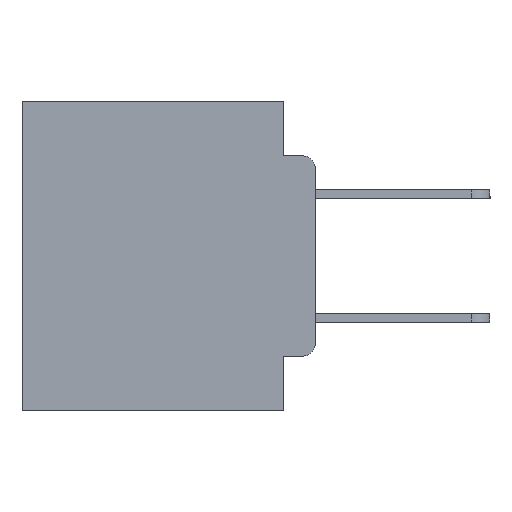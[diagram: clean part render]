
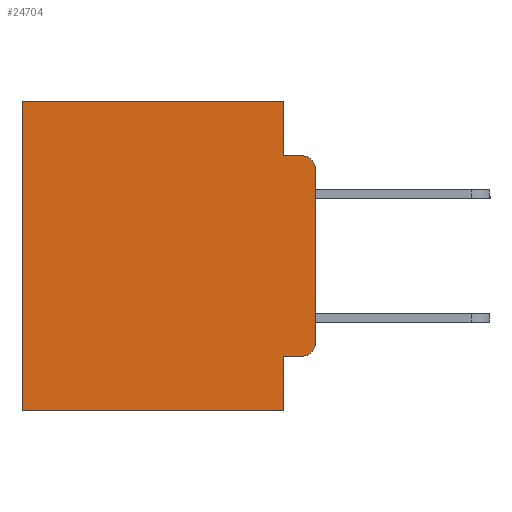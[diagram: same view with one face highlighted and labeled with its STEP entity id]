
A CAD part, left-side view. The second image highlights one B-rep face of the part: STEP entity #24704.
In plain terms, the highlighted planar face has unit normal (-1, 0, 0).
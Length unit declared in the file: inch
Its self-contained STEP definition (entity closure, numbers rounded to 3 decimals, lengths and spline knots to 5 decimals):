
#79 = CARTESIAN_POINT ( 'NONE',  ( 0.298, 0.02, -0.3915 ) ) ;
#469 = DIRECTION ( 'NONE',  ( 0., 1., 0. ) ) ;
#628 = VERTEX_POINT ( 'NONE', #25031 ) ;
#673 = ORIENTED_EDGE ( 'NONE', *, *, #13009, .T. ) ;
#2042 = VERTEX_POINT ( 'NONE', #24449 ) ;
#2286 = LINE ( 'NONE', #4082, #17867 ) ;
#2313 = DIRECTION ( 'NONE',  ( 0., 0., -1. ) ) ;
#2381 = AXIS2_PLACEMENT_3D ( 'NONE', #79, #15123, #2313 ) ;
#2742 = ORIENTED_EDGE ( 'NONE', *, *, #22740, .T. ) ;
#2755 = CARTESIAN_POINT ( 'NONE',  ( 0.298, 0.473, 0. ) ) ;
#3149 = CARTESIAN_POINT ( 'NONE',  ( 0.298, 0.051, -0.0885 ) ) ;
#3529 = VERTEX_POINT ( 'NONE', #14324 ) ;
#3605 = DIRECTION ( 'NONE',  ( 0., 0., -1. ) ) ;
#4082 = CARTESIAN_POINT ( 'NONE',  ( 0.298, 0., 0. ) ) ;
#4726 = EDGE_CURVE ( 'NONE', #12603, #23204, #25834, .T. ) ;
#5022 = AXIS2_PLACEMENT_3D ( 'NONE', #22493, #16322, #3605 ) ;
#5217 = ORIENTED_EDGE ( 'NONE', *, *, #4726, .T. ) ;
#5502 = LINE ( 'NONE', #15865, #15423 ) ;
#5717 = CARTESIAN_POINT ( 'NONE',  ( 0.298, 0.02, -0.1085 ) ) ;
#5826 = ORIENTED_EDGE ( 'NONE', *, *, #17916, .T. ) ;
#5910 = CARTESIAN_POINT ( 'NONE',  ( 0.298, 0.02, -0.0885 ) ) ;
#6348 = AXIS2_PLACEMENT_3D ( 'NONE', #5717, #20419, #8233 ) ;
#6948 = ORIENTED_EDGE ( 'NONE', *, *, #24230, .F. ) ;
#7505 = DIRECTION ( 'NONE',  ( 0., -1., 0. ) ) ;
#8233 = DIRECTION ( 'NONE',  ( 0., 0., -1. ) ) ;
#8245 = VECTOR ( 'NONE', #7505, 39.37008 ) ;
#8340 = DIRECTION ( 'NONE',  ( 0., 0., -1. ) ) ;
#8651 = ORIENTED_EDGE ( 'NONE', *, *, #15200, .F. ) ;
#8920 = VECTOR ( 'NONE', #19957, 39.37008 ) ;
#9114 = EDGE_LOOP ( 'NONE', ( #6948, #17652, #15808, #8651, #5217, #5826, #23915, #23700, #2742, #673 ) ) ;
#9290 = VERTEX_POINT ( 'NONE', #16609 ) ;
#9604 = CARTESIAN_POINT ( 'NONE',  ( 0.298, 0.473, 0. ) ) ;
#9780 = FACE_OUTER_BOUND ( 'NONE', #9114, .T. ) ;
#10179 = VECTOR ( 'NONE', #24489, 39.37008 ) ;
#10869 = CARTESIAN_POINT ( 'NONE',  ( 0.298, 0.051, -0.0885 ) ) ;
#12204 = VERTEX_POINT ( 'NONE', #5910 ) ;
#12331 = VERTEX_POINT ( 'NONE', #16849 ) ;
#12603 = VERTEX_POINT ( 'NONE', #13721 ) ;
#12658 = VECTOR ( 'NONE', #26302, 39.37008 ) ;
#13009 = EDGE_CURVE ( 'NONE', #9290, #12331, #16472, .T. ) ;
#13721 = CARTESIAN_POINT ( 'NONE',  ( 0.298, 0.051, 0. ) ) ;
#13828 = EDGE_CURVE ( 'NONE', #27100, #12204, #18033, .T. ) ;
#14053 = CARTESIAN_POINT ( 'NONE',  ( 0.298, 0.051, -0.4115 ) ) ;
#14252 = PLANE ( 'NONE',  #5022 ) ;
#14324 = CARTESIAN_POINT ( 'NONE',  ( 0.298, 0.051, -0.5 ) ) ;
#14757 = VECTOR ( 'NONE', #469, 39.37008 ) ;
#15123 = DIRECTION ( 'NONE',  ( -1., 0., 0. ) ) ;
#15200 = EDGE_CURVE ( 'NONE', #12603, #27100, #5502, .T. ) ;
#15405 = LINE ( 'NONE', #23357, #20268 ) ;
#15423 = VECTOR ( 'NONE', #17892, 39.37008 ) ;
#15744 = LINE ( 'NONE', #14053, #10179 ) ;
#15808 = ORIENTED_EDGE ( 'NONE', *, *, #13828, .F. ) ;
#15865 = CARTESIAN_POINT ( 'NONE',  ( 0.298, 0.051, 0. ) ) ;
#16322 = DIRECTION ( 'NONE',  ( 1., 0., 0. ) ) ;
#16472 = CIRCLE ( 'NONE', #2381, 0.02 ) ;
#16609 = CARTESIAN_POINT ( 'NONE',  ( 0.298, 0.02, -0.4115 ) ) ;
#16849 = CARTESIAN_POINT ( 'NONE',  ( 0.298, 0., -0.3915 ) ) ;
#17513 = CARTESIAN_POINT ( 'NONE',  ( 0.298, 0., 0. ) ) ;
#17652 = ORIENTED_EDGE ( 'NONE', *, *, #20564, .T. ) ;
#17831 = CARTESIAN_POINT ( 'NONE',  ( 0.298, 0.051, 0. ) ) ;
#17867 = VECTOR ( 'NONE', #8340, 39.37008 ) ;
#17892 = DIRECTION ( 'NONE',  ( 0., 0., -1. ) ) ;
#17916 = EDGE_CURVE ( 'NONE', #23204, #2042, #23736, .T. ) ;
#18033 = LINE ( 'NONE', #3149, #8245 ) ;
#19957 = DIRECTION ( 'NONE',  ( 0., 0., -1. ) ) ;
#20268 = VECTOR ( 'NONE', #25458, 39.37008 ) ;
#20419 = DIRECTION ( 'NONE',  ( -1., 0., 0. ) ) ;
#20564 = EDGE_CURVE ( 'NONE', #24206, #12204, #20736, .T. ) ;
#20736 = CIRCLE ( 'NONE', #6348, 0.02 ) ;
#21503 = EDGE_CURVE ( 'NONE', #628, #3529, #25583, .T. ) ;
#22493 = CARTESIAN_POINT ( 'NONE',  ( 0.298, 0., 0. ) ) ;
#22740 = EDGE_CURVE ( 'NONE', #628, #9290, #15744, .T. ) ;
#22961 = CARTESIAN_POINT ( 'NONE',  ( 0.298, 0., -0.1085 ) ) ;
#23016 = EDGE_CURVE ( 'NONE', #3529, #2042, #15405, .T. ) ;
#23204 = VERTEX_POINT ( 'NONE', #2755 ) ;
#23357 = CARTESIAN_POINT ( 'NONE',  ( 0.298, 0., -0.5 ) ) ;
#23700 = ORIENTED_EDGE ( 'NONE', *, *, #21503, .F. ) ;
#23736 = LINE ( 'NONE', #9604, #12658 ) ;
#23915 = ORIENTED_EDGE ( 'NONE', *, *, #23016, .F. ) ;
#24206 = VERTEX_POINT ( 'NONE', #22961 ) ;
#24230 = EDGE_CURVE ( 'NONE', #24206, #12331, #2286, .T. ) ;
#24449 = CARTESIAN_POINT ( 'NONE',  ( 0.298, 0.473, -0.5 ) ) ;
#24489 = DIRECTION ( 'NONE',  ( 0., -1., 0. ) ) ;
#24704 = ADVANCED_FACE ( 'NONE', ( #9780 ), #14252, .F. ) ;
#25031 = CARTESIAN_POINT ( 'NONE',  ( 0.298, 0.051, -0.4115 ) ) ;
#25458 = DIRECTION ( 'NONE',  ( 0., 1., 0. ) ) ;
#25583 = LINE ( 'NONE', #17831, #8920 ) ;
#25834 = LINE ( 'NONE', #17513, #14757 ) ;
#26302 = DIRECTION ( 'NONE',  ( 0., 0., -1. ) ) ;
#27100 = VERTEX_POINT ( 'NONE', #10869 ) ;
